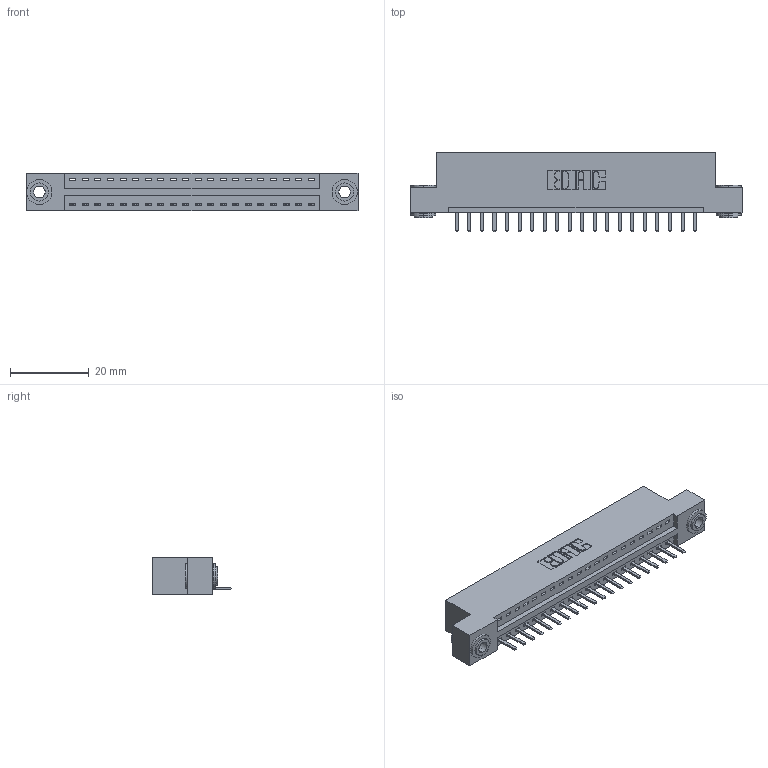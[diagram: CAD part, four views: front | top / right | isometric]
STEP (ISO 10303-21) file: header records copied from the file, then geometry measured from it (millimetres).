
FILE_DESCRIPTION (( 'STEP AP203' ), '1' );
FILE_NAME ('396-020-520-103.STEP', '2018-09-01T04:43:05', ( '' ), ( '' ), 'SwSTEP 2.0', 'SolidWorks 2016', '' );
FILE_SCHEMA (( 'CONFIG_CONTROL_DESIGN' ));
Length unit declared in the file: inch
Products named in the file (4): 345-250-002_345-250-002-102; 396-020-520-103; 346 Part_Flush Mounting Lugs - 0.156 Dia-TH; 345-292-001_345-293-120
Assembly tree (23 placements, depth 2):
  396-020-520-103
    346 Part_Flush Mounting Lugs - 0.156 Dia-TH
    345-292-001_345-293-120  x20
    345-250-002_345-250-002-102  x2
Bounding box: 84.07 x 20.02 x 9.4 mm (x, y, z)
Volume: 7858 mm3; surface area: 9611.2 mm2
Topology: 23 solids, 23 shells, 1400 faces, 4085 edges, 2666 vertices
Faces by surface type: plane 926, cylinder 466, cone 8
Entity records: 16138 total; most frequent: CARTESIAN_POINT 2763, ORIENTED_EDGE 2698, DIRECTION 2483, EDGE_CURVE 1349, LINE 1109, VECTOR 1109, VERTEX_POINT 894, AXIS2_PLACEMENT_3D 687
